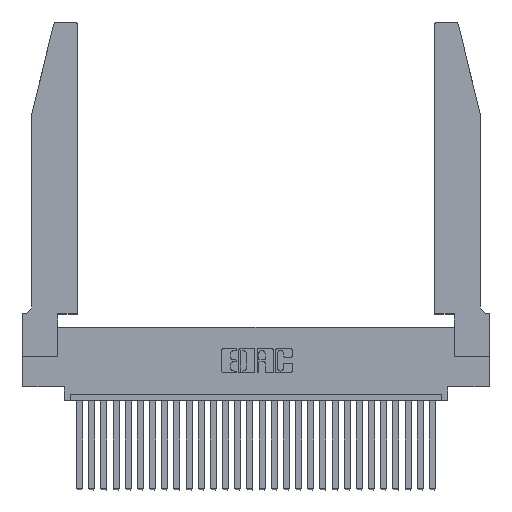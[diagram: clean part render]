
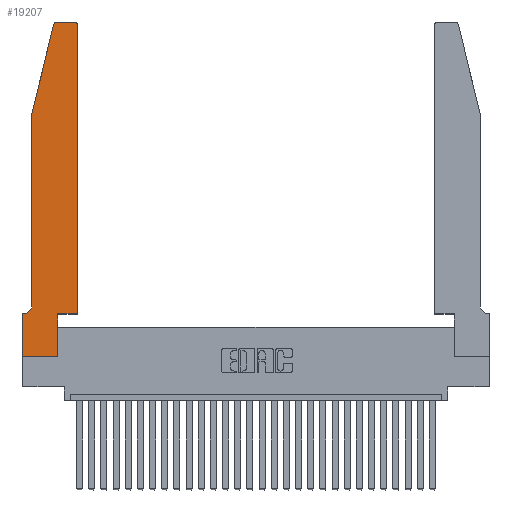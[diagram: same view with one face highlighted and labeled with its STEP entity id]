
A CAD part, top view. The second image highlights one B-rep face of the part: STEP entity #19207.
In plain terms, the highlighted planar face has unit normal (0, 0, 1).
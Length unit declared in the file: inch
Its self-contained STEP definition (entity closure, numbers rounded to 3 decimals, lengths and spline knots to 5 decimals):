
#9 = LINE ( 'NONE', #7007, #16453 ) ;
#424 = CARTESIAN_POINT ( 'NONE',  ( 0.2865, 0.35, 0.37 ) ) ;
#620 = LINE ( 'NONE', #10161, #2769 ) ;
#956 = LINE ( 'NONE', #7541, #18368 ) ;
#1017 = CARTESIAN_POINT ( 'NONE',  ( 0.284, 2.72, 0.37 ) ) ;
#1749 = EDGE_CURVE ( 'NONE', #6333, #6394, #26437, .T. ) ;
#1797 = DIRECTION ( 'NONE',  ( 0., 0., -1. ) ) ;
#1843 = DIRECTION ( 'NONE',  ( 0., -1., 0. ) ) ;
#2513 = CARTESIAN_POINT ( 'NONE',  ( 0., 0., 0.37 ) ) ;
#2558 = CARTESIAN_POINT ( 'NONE',  ( 0.4505, 0.35, 0.37 ) ) ;
#2769 = VECTOR ( 'NONE', #27969, 39.37008 ) ;
#3039 = ORIENTED_EDGE ( 'NONE', *, *, #17163, .T. ) ;
#3610 = AXIS2_PLACEMENT_3D ( 'NONE', #8900, #24521, #6859 ) ;
#4023 = EDGE_CURVE ( 'NONE', #25190, #6109, #26008, .T. ) ;
#4372 = PLANE ( 'NONE',  #3610 ) ;
#4405 = ORIENTED_EDGE ( 'NONE', *, *, #10309, .T. ) ;
#4422 = VERTEX_POINT ( 'NONE', #26867 ) ;
#4646 = AXIS2_PLACEMENT_3D ( 'NONE', #25819, #19163, #8291 ) ;
#4811 = CARTESIAN_POINT ( 'NONE',  ( 0.2865, 0., 0.37 ) ) ;
#5286 = CARTESIAN_POINT ( 'NONE',  ( 0., 0., 0.37 ) ) ;
#5395 = DIRECTION ( 'NONE',  ( 1., 0., 0. ) ) ;
#5414 = ORIENTED_EDGE ( 'NONE', *, *, #26581, .T. ) ;
#5470 = ORIENTED_EDGE ( 'NONE', *, *, #17721, .T. ) ;
#5503 = CARTESIAN_POINT ( 'NONE',  ( 0.25487, 2.72718, 0.37 ) ) ;
#5633 = CARTESIAN_POINT ( 'NONE',  ( 0.4505, 0.35, 0.37 ) ) ;
#5699 = EDGE_LOOP ( 'NONE', ( #13147, #14786, #10249, #28751, #26218, #5470, #15356, #3039, #5414, #4405, #21344, #20005 ) ) ;
#6109 = VERTEX_POINT ( 'NONE', #5503 ) ;
#6333 = VERTEX_POINT ( 'NONE', #21458 ) ;
#6377 = FACE_OUTER_BOUND ( 'NONE', #5699, .T. ) ;
#6394 = VERTEX_POINT ( 'NONE', #10040 ) ;
#6859 = DIRECTION ( 'NONE',  ( 1., 0., 0. ) ) ;
#7007 = CARTESIAN_POINT ( 'NONE',  ( 0.2605, 2.75, 0.37 ) ) ;
#7541 = CARTESIAN_POINT ( 'NONE',  ( 0.4505, 0.35, 0.37 ) ) ;
#7618 = VECTOR ( 'NONE', #1843, 39.37008 ) ;
#7662 = LINE ( 'NONE', #5286, #24761 ) ;
#7800 = VECTOR ( 'NONE', #18614, 39.37008 ) ;
#8066 = LINE ( 'NONE', #2558, #27927 ) ;
#8291 = DIRECTION ( 'NONE',  ( 1., 0., 0. ) ) ;
#8795 = VERTEX_POINT ( 'NONE', #12269 ) ;
#8900 = CARTESIAN_POINT ( 'NONE',  ( 0., 0.35, 0.37 ) ) ;
#8901 = EDGE_CURVE ( 'NONE', #15955, #21479, #27322, .T. ) ;
#9341 = LINE ( 'NONE', #21739, #7618 ) ;
#10040 = CARTESIAN_POINT ( 'NONE',  ( 0.0055, 0.35, 0.37 ) ) ;
#10161 = CARTESIAN_POINT ( 'NONE',  ( 0.0755, 0.35, 0.37 ) ) ;
#10249 = ORIENTED_EDGE ( 'NONE', *, *, #14213, .T. ) ;
#10309 = EDGE_CURVE ( 'NONE', #13181, #10872, #8066, .T. ) ;
#10438 = EDGE_CURVE ( 'NONE', #4422, #25190, #9, .T. ) ;
#10492 = DIRECTION ( 'NONE',  ( -1., 0., 0. ) ) ;
#10614 = VECTOR ( 'NONE', #14100, 39.37008 ) ;
#10872 = VERTEX_POINT ( 'NONE', #5633 ) ;
#12269 = CARTESIAN_POINT ( 'NONE',  ( 0.4505, 2.72, 0.37 ) ) ;
#13147 = ORIENTED_EDGE ( 'NONE', *, *, #10438, .T. ) ;
#13181 = VERTEX_POINT ( 'NONE', #16593 ) ;
#13619 = VERTEX_POINT ( 'NONE', #4811 ) ;
#14100 = DIRECTION ( 'NONE',  ( 0., -1., 0. ) ) ;
#14205 = AXIS2_PLACEMENT_3D ( 'NONE', #1017, #16658, #18852 ) ;
#14213 = EDGE_CURVE ( 'NONE', #6109, #14780, #19974, .T. ) ;
#14780 = VERTEX_POINT ( 'NONE', #27822 ) ;
#14786 = ORIENTED_EDGE ( 'NONE', *, *, #4023, .T. ) ;
#15356 = ORIENTED_EDGE ( 'NONE', *, *, #8901, .T. ) ;
#15955 = VERTEX_POINT ( 'NONE', #20307 ) ;
#16157 = CARTESIAN_POINT ( 'NONE',  ( 0.284, 2.75, 0.37 ) ) ;
#16231 = LINE ( 'NONE', #424, #22456 ) ;
#16453 = VECTOR ( 'NONE', #22401, 39.37008 ) ;
#16593 = CARTESIAN_POINT ( 'NONE',  ( 0.2865, 0.35, 0.37 ) ) ;
#16658 = DIRECTION ( 'NONE',  ( 0., 0., 1. ) ) ;
#17163 = EDGE_CURVE ( 'NONE', #21479, #13619, #7662, .T. ) ;
#17721 = EDGE_CURVE ( 'NONE', #6394, #15955, #620, .T. ) ;
#18034 = EDGE_CURVE ( 'NONE', #14780, #6333, #9341, .T. ) ;
#18368 = VECTOR ( 'NONE', #23157, 39.37008 ) ;
#18459 = DIRECTION ( 'NONE',  ( 0., 1., 0. ) ) ;
#18510 = CARTESIAN_POINT ( 'NONE',  ( 0.0755, 2., 0.37 ) ) ;
#18614 = DIRECTION ( 'NONE',  ( -0.239, -0.971, 0. ) ) ;
#18852 = DIRECTION ( 'NONE',  ( 1., 0., 0. ) ) ;
#19163 = DIRECTION ( 'NONE',  ( 0., 0., 1. ) ) ;
#19207 = ADVANCED_FACE ( 'NONE', ( #6377 ), #4372, .T. ) ;
#19698 = CIRCLE ( 'NONE', #4646, 0.03 ) ;
#19974 = LINE ( 'NONE', #18510, #7800 ) ;
#20005 = ORIENTED_EDGE ( 'NONE', *, *, #26050, .T. ) ;
#20307 = CARTESIAN_POINT ( 'NONE',  ( 0., 0.35, 0.37 ) ) ;
#20505 = DIRECTION ( 'NONE',  ( 1., 0., 0. ) ) ;
#20654 = AXIS2_PLACEMENT_3D ( 'NONE', #23861, #1797, #10492 ) ;
#21344 = ORIENTED_EDGE ( 'NONE', *, *, #22277, .T. ) ;
#21458 = CARTESIAN_POINT ( 'NONE',  ( 0.0755, 0.42, 0.37 ) ) ;
#21479 = VERTEX_POINT ( 'NONE', #2513 ) ;
#21739 = CARTESIAN_POINT ( 'NONE',  ( 0.0755, 2., 0.37 ) ) ;
#22277 = EDGE_CURVE ( 'NONE', #10872, #8795, #956, .T. ) ;
#22401 = DIRECTION ( 'NONE',  ( -1., 0., 0. ) ) ;
#22456 = VECTOR ( 'NONE', #18459, 39.37008 ) ;
#23157 = DIRECTION ( 'NONE',  ( 0., 1., 0. ) ) ;
#23861 = CARTESIAN_POINT ( 'NONE',  ( 0.0055, 0.42, 0.37 ) ) ;
#24521 = DIRECTION ( 'NONE',  ( 0., 0., 1. ) ) ;
#24761 = VECTOR ( 'NONE', #5395, 39.37008 ) ;
#24908 = CARTESIAN_POINT ( 'NONE',  ( 0., 0., 0.37 ) ) ;
#25190 = VERTEX_POINT ( 'NONE', #16157 ) ;
#25819 = CARTESIAN_POINT ( 'NONE',  ( 0.4205, 2.72, 0.37 ) ) ;
#26008 = CIRCLE ( 'NONE', #14205, 0.03 ) ;
#26050 = EDGE_CURVE ( 'NONE', #8795, #4422, #19698, .T. ) ;
#26218 = ORIENTED_EDGE ( 'NONE', *, *, #1749, .T. ) ;
#26437 = CIRCLE ( 'NONE', #20654, 0.07 ) ;
#26581 = EDGE_CURVE ( 'NONE', #13619, #13181, #16231, .T. ) ;
#26867 = CARTESIAN_POINT ( 'NONE',  ( 0.4205, 2.75, 0.37 ) ) ;
#27322 = LINE ( 'NONE', #24908, #10614 ) ;
#27822 = CARTESIAN_POINT ( 'NONE',  ( 0.0755, 2., 0.37 ) ) ;
#27927 = VECTOR ( 'NONE', #20505, 39.37008 ) ;
#27969 = DIRECTION ( 'NONE',  ( -1., 0., 0. ) ) ;
#28751 = ORIENTED_EDGE ( 'NONE', *, *, #18034, .T. ) ;
